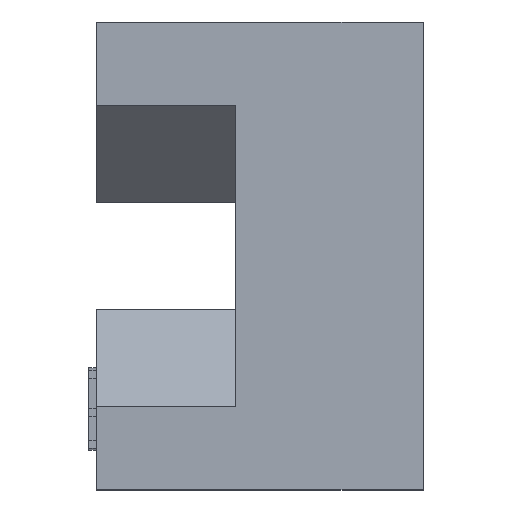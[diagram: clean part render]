
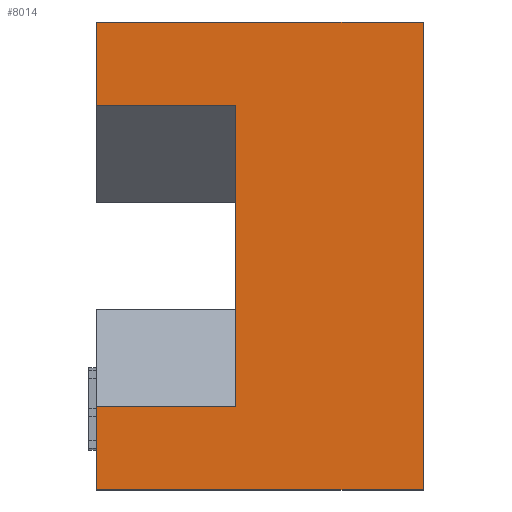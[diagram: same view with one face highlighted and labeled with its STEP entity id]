
A CAD part, left-side view. The second image highlights one B-rep face of the part: STEP entity #8014.
In plain terms, the highlighted planar face has unit normal (-1, 0, 0).
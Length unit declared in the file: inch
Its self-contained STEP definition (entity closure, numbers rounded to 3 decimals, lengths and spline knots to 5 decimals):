
#218 = LINE ( 'NONE', #14344, #1339 ) ;
#274 = EDGE_CURVE ( 'NONE', #12827, #7292, #10889, .T. ) ;
#354 = EDGE_LOOP ( 'NONE', ( #2541, #10142, #10980, #1972, #14522, #6322, #5969, #10904 ) ) ;
#373 = DIRECTION ( 'NONE',  ( 0., 0., 1. ) ) ;
#595 = CARTESIAN_POINT ( 'NONE',  ( -4.5, 0.218, -0.156 ) ) ;
#747 = FACE_OUTER_BOUND ( 'NONE', #354, .T. ) ;
#817 = CARTESIAN_POINT ( 'NONE',  ( -4.5, 0., 0.156 ) ) ;
#818 = DIRECTION ( 'NONE',  ( 1., 0., 0. ) ) ;
#1339 = VECTOR ( 'NONE', #6276, 39.37008 ) ;
#1551 = AXIS2_PLACEMENT_3D ( 'NONE', #595, #818, #5296 ) ;
#1641 = CARTESIAN_POINT ( 'NONE',  ( -4.5, 0.125, -0.1005 ) ) ;
#1972 = ORIENTED_EDGE ( 'NONE', *, *, #4561, .T. ) ;
#1989 = LINE ( 'NONE', #2861, #9943 ) ;
#2136 = VERTEX_POINT ( 'NONE', #4221 ) ;
#2224 = VERTEX_POINT ( 'NONE', #817 ) ;
#2260 = CARTESIAN_POINT ( 'NONE',  ( -4.5, 0.125, -0.1005 ) ) ;
#2366 = VECTOR ( 'NONE', #13221, 39.37008 ) ;
#2541 = ORIENTED_EDGE ( 'NONE', *, *, #13785, .F. ) ;
#2861 = CARTESIAN_POINT ( 'NONE',  ( -4.5, 0.218, -0.156 ) ) ;
#2901 = VECTOR ( 'NONE', #3780, 39.37008 ) ;
#2978 = LINE ( 'NONE', #9805, #8540 ) ;
#3124 = CARTESIAN_POINT ( 'NONE',  ( -4.5, 0.125, 0.1005 ) ) ;
#3186 = VERTEX_POINT ( 'NONE', #3124 ) ;
#3780 = DIRECTION ( 'NONE',  ( 0., 0., 1. ) ) ;
#3947 = DIRECTION ( 'NONE',  ( 0., -1., 0. ) ) ;
#4093 = LINE ( 'NONE', #8456, #2366 ) ;
#4221 = CARTESIAN_POINT ( 'NONE',  ( -4.5, 0.218, -0.1005 ) ) ;
#4464 = LINE ( 'NONE', #1641, #8408 ) ;
#4561 = EDGE_CURVE ( 'NONE', #7407, #13898, #13147, .T. ) ;
#5146 = VECTOR ( 'NONE', #373, 39.37008 ) ;
#5283 = DIRECTION ( 'NONE',  ( 0., 1., 0. ) ) ;
#5296 = DIRECTION ( 'NONE',  ( 0., 0., -1. ) ) ;
#5672 = EDGE_CURVE ( 'NONE', #13898, #2224, #13211, .T. ) ;
#5969 = ORIENTED_EDGE ( 'NONE', *, *, #274, .F. ) ;
#6276 = DIRECTION ( 'NONE',  ( 0., -1., 0. ) ) ;
#6322 = ORIENTED_EDGE ( 'NONE', *, *, #14378, .F. ) ;
#7292 = VERTEX_POINT ( 'NONE', #9851 ) ;
#7407 = VERTEX_POINT ( 'NONE', #14691 ) ;
#8014 = ADVANCED_FACE ( 'NONE', ( #747 ), #11199, .F. ) ;
#8037 = DIRECTION ( 'NONE',  ( 0., 0., 1. ) ) ;
#8289 = CARTESIAN_POINT ( 'NONE',  ( -4.5, 0., -0.156 ) ) ;
#8300 = CARTESIAN_POINT ( 'NONE',  ( -4.5, 0., -0.156 ) ) ;
#8408 = VECTOR ( 'NONE', #14543, 39.37008 ) ;
#8456 = CARTESIAN_POINT ( 'NONE',  ( -4.5, 0.125, -0.1005 ) ) ;
#8540 = VECTOR ( 'NONE', #5283, 39.37008 ) ;
#8674 = EDGE_CURVE ( 'NONE', #12630, #2136, #4464, .T. ) ;
#9342 = EDGE_CURVE ( 'NONE', #3186, #12827, #2978, .T. ) ;
#9516 = CARTESIAN_POINT ( 'NONE',  ( -4.5, 0.218, -0.156 ) ) ;
#9694 = CARTESIAN_POINT ( 'NONE',  ( -4.5, 0.218, -0.156 ) ) ;
#9805 = CARTESIAN_POINT ( 'NONE',  ( -4.5, 0.125, 0.1005 ) ) ;
#9851 = CARTESIAN_POINT ( 'NONE',  ( -4.5, 0.218, 0.156 ) ) ;
#9943 = VECTOR ( 'NONE', #8037, 39.37008 ) ;
#10142 = ORIENTED_EDGE ( 'NONE', *, *, #8674, .T. ) ;
#10528 = VECTOR ( 'NONE', #3947, 39.37008 ) ;
#10889 = LINE ( 'NONE', #9516, #5146 ) ;
#10904 = ORIENTED_EDGE ( 'NONE', *, *, #9342, .F. ) ;
#10980 = ORIENTED_EDGE ( 'NONE', *, *, #12039, .F. ) ;
#11199 = PLANE ( 'NONE',  #1551 ) ;
#11217 = CARTESIAN_POINT ( 'NONE',  ( -4.5, 0.218, 0.1005 ) ) ;
#12039 = EDGE_CURVE ( 'NONE', #7407, #2136, #1989, .T. ) ;
#12630 = VERTEX_POINT ( 'NONE', #2260 ) ;
#12827 = VERTEX_POINT ( 'NONE', #11217 ) ;
#13147 = LINE ( 'NONE', #9694, #10528 ) ;
#13211 = LINE ( 'NONE', #8300, #2901 ) ;
#13221 = DIRECTION ( 'NONE',  ( 0., 0., 1. ) ) ;
#13785 = EDGE_CURVE ( 'NONE', #12630, #3186, #4093, .T. ) ;
#13898 = VERTEX_POINT ( 'NONE', #8289 ) ;
#14344 = CARTESIAN_POINT ( 'NONE',  ( -4.5, 0.218, 0.156 ) ) ;
#14378 = EDGE_CURVE ( 'NONE', #7292, #2224, #218, .T. ) ;
#14522 = ORIENTED_EDGE ( 'NONE', *, *, #5672, .T. ) ;
#14543 = DIRECTION ( 'NONE',  ( 0., 1., 0. ) ) ;
#14691 = CARTESIAN_POINT ( 'NONE',  ( -4.5, 0.218, -0.156 ) ) ;
